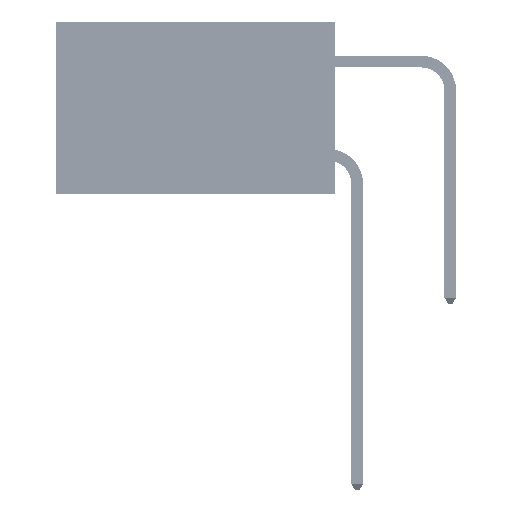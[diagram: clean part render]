
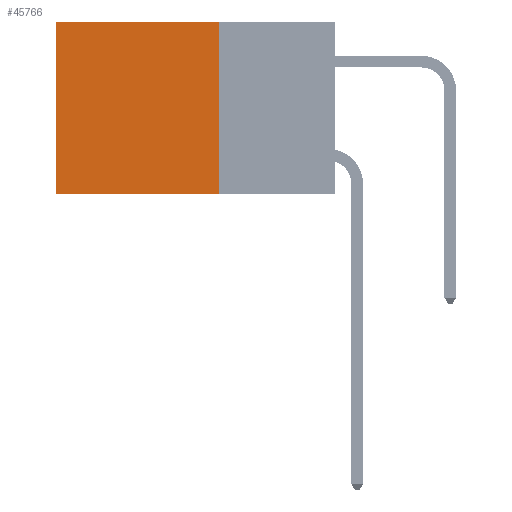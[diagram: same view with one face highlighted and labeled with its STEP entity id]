
A CAD part, left-side view. The second image highlights one B-rep face of the part: STEP entity #45766.
In plain terms, the highlighted planar face has unit normal (-1, 0, 0).
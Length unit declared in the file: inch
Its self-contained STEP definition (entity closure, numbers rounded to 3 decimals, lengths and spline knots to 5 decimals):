
#1362 = DIRECTION ( 'NONE',  ( 0., 1., 0. ) ) ;
#1674 = VERTEX_POINT ( 'NONE', #13301 ) ;
#1813 = LINE ( 'NONE', #4710, #42506 ) ;
#2950 = DIRECTION ( 'NONE',  ( 0., 0., -1. ) ) ;
#3364 = DIRECTION ( 'NONE',  ( 0., 0., -1. ) ) ;
#4036 = ORIENTED_EDGE ( 'NONE', *, *, #10757, .F. ) ;
#4710 = CARTESIAN_POINT ( 'NONE',  ( 0.2875, 0.25, -0.37 ) ) ;
#6359 = CARTESIAN_POINT ( 'NONE',  ( 0.2875, 0.6, 0. ) ) ;
#6970 = CARTESIAN_POINT ( 'NONE',  ( 0.2875, 0.25, 0. ) ) ;
#8189 = VECTOR ( 'NONE', #12925, 39.37008 ) ;
#9672 = FACE_OUTER_BOUND ( 'NONE', #17456, .T. ) ;
#10392 = CARTESIAN_POINT ( 'NONE',  ( 0.2875, 0.6, 0. ) ) ;
#10757 = EDGE_CURVE ( 'NONE', #30256, #1674, #13952, .T. ) ;
#11656 = VECTOR ( 'NONE', #3364, 39.37008 ) ;
#12925 = DIRECTION ( 'NONE',  ( 0., 0., -1. ) ) ;
#13291 = DIRECTION ( 'NONE',  ( 0., 1., 0. ) ) ;
#13301 = CARTESIAN_POINT ( 'NONE',  ( 0.2875, 0.25, -0.37 ) ) ;
#13381 = VERTEX_POINT ( 'NONE', #23146 ) ;
#13952 = LINE ( 'NONE', #6970, #11656 ) ;
#15174 = ORIENTED_EDGE ( 'NONE', *, *, #38271, .F. ) ;
#17456 = EDGE_LOOP ( 'NONE', ( #45266, #15174, #4036, #35209 ) ) ;
#17653 = CARTESIAN_POINT ( 'NONE',  ( 0.2875, 0.25, 0. ) ) ;
#21328 = VERTEX_POINT ( 'NONE', #10392 ) ;
#22548 = VECTOR ( 'NONE', #13291, 39.37008 ) ;
#23146 = CARTESIAN_POINT ( 'NONE',  ( 0.2875, 0.6, -0.37 ) ) ;
#28610 = CARTESIAN_POINT ( 'NONE',  ( 0.2875, 0.25, 0. ) ) ;
#30100 = LINE ( 'NONE', #44744, #22548 ) ;
#30256 = VERTEX_POINT ( 'NONE', #17653 ) ;
#31514 = DIRECTION ( 'NONE',  ( 1., 0., 0. ) ) ;
#31736 = EDGE_CURVE ( 'NONE', #30256, #21328, #30100, .T. ) ;
#35209 = ORIENTED_EDGE ( 'NONE', *, *, #31736, .T. ) ;
#35821 = PLANE ( 'NONE',  #45640 ) ;
#38271 = EDGE_CURVE ( 'NONE', #1674, #13381, #1813, .T. ) ;
#42506 = VECTOR ( 'NONE', #1362, 39.37008 ) ;
#44744 = CARTESIAN_POINT ( 'NONE',  ( 0.2875, 0.25, 0. ) ) ;
#45266 = ORIENTED_EDGE ( 'NONE', *, *, #47297, .T. ) ;
#45640 = AXIS2_PLACEMENT_3D ( 'NONE', #28610, #31514, #2950 ) ;
#45766 = ADVANCED_FACE ( 'NONE', ( #9672 ), #35821, .F. ) ;
#45812 = LINE ( 'NONE', #6359, #8189 ) ;
#47297 = EDGE_CURVE ( 'NONE', #21328, #13381, #45812, .T. ) ;
